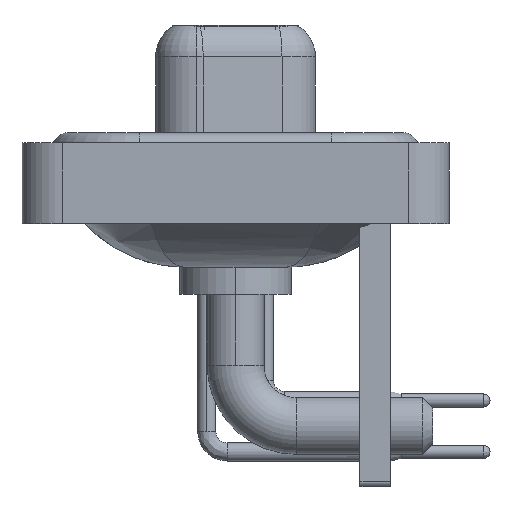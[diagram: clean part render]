
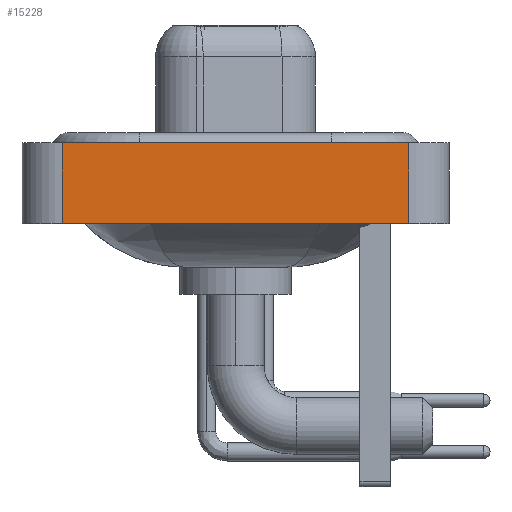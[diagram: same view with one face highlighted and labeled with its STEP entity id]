
A CAD part, left-side view. The second image highlights one B-rep face of the part: STEP entity #15228.
In plain terms, the highlighted planar face has unit normal (-1, 0, 0).
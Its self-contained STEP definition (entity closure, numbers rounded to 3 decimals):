
#633 = LINE ( 'NONE', #7222, #16071 ) ;
#1870 = ORIENTED_EDGE ( 'NONE', *, *, #5349, .F. ) ;
#2030 = DIRECTION ( 'NONE',  ( 0., 0., 1. ) ) ;
#2185 = CARTESIAN_POINT ( 'NONE',  ( -7.3, -8.55, 0.4 ) ) ;
#2353 = DIRECTION ( 'NONE',  ( -1., 0., 0. ) ) ;
#2587 = CARTESIAN_POINT ( 'NONE',  ( -7.3, -8.55, -3.6 ) ) ;
#3505 = ORIENTED_EDGE ( 'NONE', *, *, #20444, .T. ) ;
#3702 = EDGE_LOOP ( 'NONE', ( #13472, #13517, #1870, #3505 ) ) ;
#3738 = CARTESIAN_POINT ( 'NONE',  ( -7.3, -8.55, -3.6 ) ) ;
#5349 = EDGE_CURVE ( 'NONE', #16667, #15154, #13486, .T. ) ;
#5495 = FACE_OUTER_BOUND ( 'NONE', #3702, .T. ) ;
#5727 = PLANE ( 'NONE',  #16457 ) ;
#5921 = VECTOR ( 'NONE', #19047, 1000. ) ;
#6794 = CARTESIAN_POINT ( 'NONE',  ( -7.3, -8.55, -3.6 ) ) ;
#7222 = CARTESIAN_POINT ( 'NONE',  ( -7.3, -8.55, 0.4 ) ) ;
#8523 = VERTEX_POINT ( 'NONE', #2185 ) ;
#9633 = EDGE_CURVE ( 'NONE', #10838, #8523, #19464, .T. ) ;
#10334 = DIRECTION ( 'NONE',  ( 0., 0., 1. ) ) ;
#10729 = VECTOR ( 'NONE', #10334, 1000. ) ;
#10838 = VERTEX_POINT ( 'NONE', #6794 ) ;
#11624 = DIRECTION ( 'NONE',  ( 0., -1., 0. ) ) ;
#11749 = DIRECTION ( 'NONE',  ( 0., -1., 0. ) ) ;
#12312 = CARTESIAN_POINT ( 'NONE',  ( -7.3, -8.55, -3.6 ) ) ;
#13472 = ORIENTED_EDGE ( 'NONE', *, *, #9633, .T. ) ;
#13486 = LINE ( 'NONE', #13594, #10729 ) ;
#13517 = ORIENTED_EDGE ( 'NONE', *, *, #18616, .F. ) ;
#13594 = CARTESIAN_POINT ( 'NONE',  ( -7.3, 8.55, -3.6 ) ) ;
#15154 = VERTEX_POINT ( 'NONE', #18061 ) ;
#15228 = ADVANCED_FACE ( 'NONE', ( #5495 ), #5727, .T. ) ;
#15301 = LINE ( 'NONE', #3738, #15309 ) ;
#15309 = VECTOR ( 'NONE', #11624, 1000. ) ;
#16071 = VECTOR ( 'NONE', #11749, 1000. ) ;
#16457 = AXIS2_PLACEMENT_3D ( 'NONE', #12312, #2353, #2030 ) ;
#16667 = VERTEX_POINT ( 'NONE', #19442 ) ;
#18061 = CARTESIAN_POINT ( 'NONE',  ( -7.3, 8.55, 0.4 ) ) ;
#18616 = EDGE_CURVE ( 'NONE', #15154, #8523, #633, .T. ) ;
#19047 = DIRECTION ( 'NONE',  ( 0., 0., 1. ) ) ;
#19442 = CARTESIAN_POINT ( 'NONE',  ( -7.3, 8.55, -3.6 ) ) ;
#19464 = LINE ( 'NONE', #2587, #5921 ) ;
#20444 = EDGE_CURVE ( 'NONE', #16667, #10838, #15301, .T. ) ;
